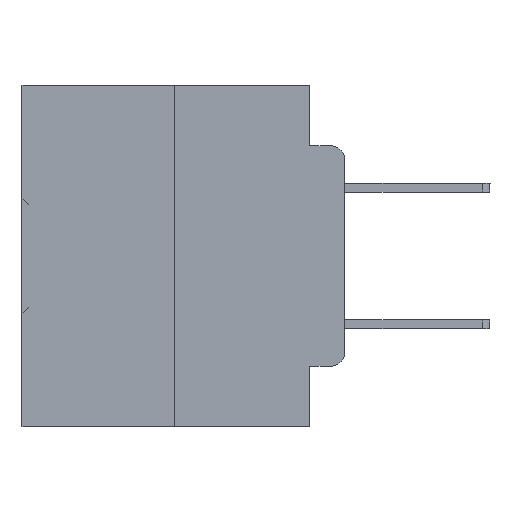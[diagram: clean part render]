
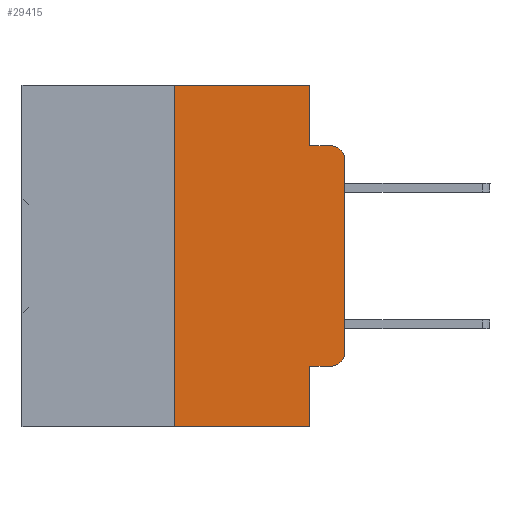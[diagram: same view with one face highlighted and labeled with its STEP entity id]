
A CAD part, left-side view. The second image highlights one B-rep face of the part: STEP entity #29415.
In plain terms, the highlighted planar face has unit normal (-1, 0, 0).
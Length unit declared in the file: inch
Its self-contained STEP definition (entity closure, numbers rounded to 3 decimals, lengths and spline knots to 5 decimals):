
#95 = CIRCLE ( 'NONE', #33086, 0.02 ) ;
#214 = EDGE_CURVE ( 'NONE', #16679, #8727, #25533, .T. ) ;
#228 = VERTEX_POINT ( 'NONE', #4334 ) ;
#1520 = EDGE_CURVE ( 'NONE', #18888, #23718, #19950, .T. ) ;
#2291 = CARTESIAN_POINT ( 'NONE',  ( 0., 0.02, -0.1085 ) ) ;
#2356 = CARTESIAN_POINT ( 'NONE',  ( 0., 0., -0.3915 ) ) ;
#2416 = DIRECTION ( 'NONE',  ( -1., 0., 0. ) ) ;
#2560 = VERTEX_POINT ( 'NONE', #22864 ) ;
#2618 = DIRECTION ( 'NONE',  ( 0., -1., 0. ) ) ;
#3550 = DIRECTION ( 'NONE',  ( 0., -1., 0. ) ) ;
#3842 = ORIENTED_EDGE ( 'NONE', *, *, #30016, .F. ) ;
#4094 = CARTESIAN_POINT ( 'NONE',  ( 0., 0.051, 0. ) ) ;
#4334 = CARTESIAN_POINT ( 'NONE',  ( 0., 0.25, 0. ) ) ;
#4675 = CARTESIAN_POINT ( 'NONE',  ( 0., 0.25, -0.5 ) ) ;
#4856 = CARTESIAN_POINT ( 'NONE',  ( 0., 0.02, -0.3915 ) ) ;
#4882 = LINE ( 'NONE', #5166, #8563 ) ;
#5166 = CARTESIAN_POINT ( 'NONE',  ( 0., 0.473, -0.5 ) ) ;
#5551 = CARTESIAN_POINT ( 'NONE',  ( 0., 0.25, 0. ) ) ;
#7322 = VECTOR ( 'NONE', #31178, 39.37008 ) ;
#7551 = VERTEX_POINT ( 'NONE', #24552 ) ;
#7560 = VECTOR ( 'NONE', #19896, 39.37008 ) ;
#7852 = EDGE_CURVE ( 'NONE', #12517, #2560, #4882, .T. ) ;
#8277 = DIRECTION ( 'NONE',  ( 0., 0., -1. ) ) ;
#8563 = VECTOR ( 'NONE', #2618, 39.37008 ) ;
#8686 = CARTESIAN_POINT ( 'NONE',  ( 0., 0., -0.1085 ) ) ;
#8727 = VERTEX_POINT ( 'NONE', #32290 ) ;
#8874 = EDGE_CURVE ( 'NONE', #7551, #2560, #36267, .T. ) ;
#8880 = CARTESIAN_POINT ( 'NONE',  ( 0., 0.051, -0.4115 ) ) ;
#9645 = ORIENTED_EDGE ( 'NONE', *, *, #13278, .T. ) ;
#9723 = ORIENTED_EDGE ( 'NONE', *, *, #30834, .F. ) ;
#9931 = VECTOR ( 'NONE', #22258, 39.37008 ) ;
#10887 = DIRECTION ( 'NONE',  ( 0., 0., -1. ) ) ;
#12215 = EDGE_CURVE ( 'NONE', #228, #22611, #27814, .T. ) ;
#12517 = VERTEX_POINT ( 'NONE', #4675 ) ;
#13276 = CARTESIAN_POINT ( 'NONE',  ( 0., 0.051, -0.0885 ) ) ;
#13278 = EDGE_CURVE ( 'NONE', #7551, #21314, #31835, .T. ) ;
#13530 = AXIS2_PLACEMENT_3D ( 'NONE', #19652, #37621, #17124 ) ;
#14806 = VECTOR ( 'NONE', #29205, 39.37008 ) ;
#16679 = VERTEX_POINT ( 'NONE', #31340 ) ;
#17124 = DIRECTION ( 'NONE',  ( 0., 0., -1. ) ) ;
#17364 = VECTOR ( 'NONE', #3550, 39.37008 ) ;
#17578 = EDGE_CURVE ( 'NONE', #21314, #18888, #22167, .T. ) ;
#18422 = DIRECTION ( 'NONE',  ( 0., -1., 0. ) ) ;
#18888 = VERTEX_POINT ( 'NONE', #2356 ) ;
#19334 = CARTESIAN_POINT ( 'NONE',  ( 0., 0., 0. ) ) ;
#19652 = CARTESIAN_POINT ( 'NONE',  ( 0., 0.473, 0. ) ) ;
#19839 = LINE ( 'NONE', #5551, #14806 ) ;
#19896 = DIRECTION ( 'NONE',  ( 0., 0., -1. ) ) ;
#19950 = LINE ( 'NONE', #19334, #9931 ) ;
#20163 = EDGE_LOOP ( 'NONE', ( #20331, #28659, #36743, #3842, #28842, #9723, #31390, #22816, #9645, #25836 ) ) ;
#20331 = ORIENTED_EDGE ( 'NONE', *, *, #1520, .T. ) ;
#20465 = VECTOR ( 'NONE', #18422, 39.37008 ) ;
#21314 = VERTEX_POINT ( 'NONE', #33211 ) ;
#21966 = LINE ( 'NONE', #25223, #7322 ) ;
#22167 = CIRCLE ( 'NONE', #33535, 0.02 ) ;
#22258 = DIRECTION ( 'NONE',  ( 0., 0., 1. ) ) ;
#22611 = VERTEX_POINT ( 'NONE', #4094 ) ;
#22816 = ORIENTED_EDGE ( 'NONE', *, *, #8874, .F. ) ;
#22864 = CARTESIAN_POINT ( 'NONE',  ( 0., 0.051, -0.5 ) ) ;
#23718 = VERTEX_POINT ( 'NONE', #8686 ) ;
#24552 = CARTESIAN_POINT ( 'NONE',  ( 0., 0.051, -0.4115 ) ) ;
#25223 = CARTESIAN_POINT ( 'NONE',  ( 0., 0.051, 0. ) ) ;
#25533 = LINE ( 'NONE', #13276, #36013 ) ;
#25836 = ORIENTED_EDGE ( 'NONE', *, *, #17578, .T. ) ;
#27814 = LINE ( 'NONE', #35051, #17364 ) ;
#28659 = ORIENTED_EDGE ( 'NONE', *, *, #33115, .T. ) ;
#28842 = ORIENTED_EDGE ( 'NONE', *, *, #12215, .F. ) ;
#29205 = DIRECTION ( 'NONE',  ( 0., 0., 1. ) ) ;
#29415 = ADVANCED_FACE ( 'NONE', ( #30517 ), #34442, .F. ) ;
#30016 = EDGE_CURVE ( 'NONE', #22611, #16679, #21966, .T. ) ;
#30517 = FACE_OUTER_BOUND ( 'NONE', #20163, .T. ) ;
#30834 = EDGE_CURVE ( 'NONE', #12517, #228, #19839, .T. ) ;
#31178 = DIRECTION ( 'NONE',  ( 0., 0., -1. ) ) ;
#31226 = DIRECTION ( 'NONE',  ( -1., 0., 0. ) ) ;
#31340 = CARTESIAN_POINT ( 'NONE',  ( 0., 0.051, -0.0885 ) ) ;
#31390 = ORIENTED_EDGE ( 'NONE', *, *, #7852, .T. ) ;
#31835 = LINE ( 'NONE', #8880, #20465 ) ;
#32290 = CARTESIAN_POINT ( 'NONE',  ( 0., 0.02, -0.0885 ) ) ;
#33086 = AXIS2_PLACEMENT_3D ( 'NONE', #2291, #2416, #8277 ) ;
#33115 = EDGE_CURVE ( 'NONE', #23718, #8727, #95, .T. ) ;
#33211 = CARTESIAN_POINT ( 'NONE',  ( 0., 0.02, -0.4115 ) ) ;
#33535 = AXIS2_PLACEMENT_3D ( 'NONE', #4856, #31226, #10887 ) ;
#34357 = CARTESIAN_POINT ( 'NONE',  ( 0., 0.051, 0. ) ) ;
#34442 = PLANE ( 'NONE',  #13530 ) ;
#35051 = CARTESIAN_POINT ( 'NONE',  ( 0., 0.473, 0. ) ) ;
#36013 = VECTOR ( 'NONE', #36595, 39.37008 ) ;
#36267 = LINE ( 'NONE', #34357, #7560 ) ;
#36595 = DIRECTION ( 'NONE',  ( 0., -1., 0. ) ) ;
#36743 = ORIENTED_EDGE ( 'NONE', *, *, #214, .F. ) ;
#37621 = DIRECTION ( 'NONE',  ( 1., 0., 0. ) ) ;
